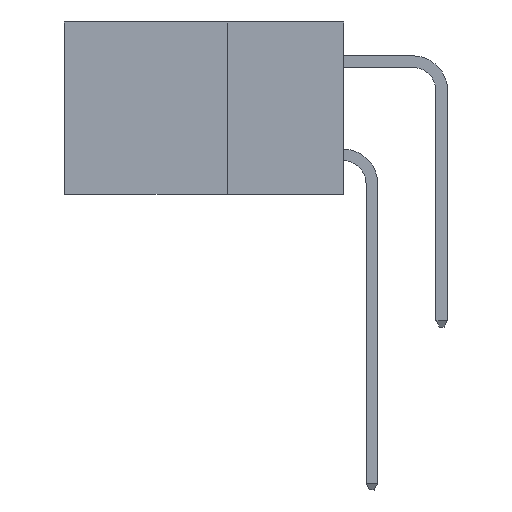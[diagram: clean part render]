
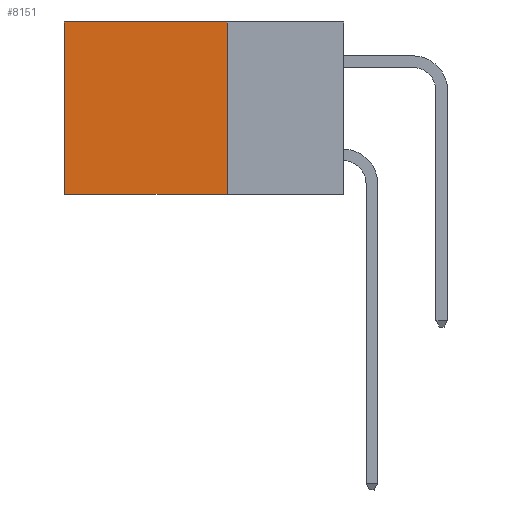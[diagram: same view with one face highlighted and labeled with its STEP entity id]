
A CAD part, left-side view. The second image highlights one B-rep face of the part: STEP entity #8151.
In plain terms, the highlighted planar face has unit normal (-1, 0, 0).
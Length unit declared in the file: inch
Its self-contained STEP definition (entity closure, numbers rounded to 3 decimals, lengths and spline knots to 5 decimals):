
#38 = VERTEX_POINT ( 'NONE', #597 ) ;
#238 = FACE_OUTER_BOUND ( 'NONE', #12392, .T. ) ;
#333 = LINE ( 'NONE', #8152, #9993 ) ;
#480 = CARTESIAN_POINT ( 'NONE',  ( 0.298, 0.6, 0. ) ) ;
#597 = CARTESIAN_POINT ( 'NONE',  ( 0.298, 0.6, -0.37 ) ) ;
#1144 = CARTESIAN_POINT ( 'NONE',  ( 0.298, 0.25, 0. ) ) ;
#1227 = VERTEX_POINT ( 'NONE', #12031 ) ;
#2261 = PLANE ( 'NONE',  #10365 ) ;
#2328 = VERTEX_POINT ( 'NONE', #14279 ) ;
#2749 = VERTEX_POINT ( 'NONE', #480 ) ;
#3270 = EDGE_CURVE ( 'NONE', #1227, #2328, #13689, .T. ) ;
#5617 = DIRECTION ( 'NONE',  ( 0., 0., -1. ) ) ;
#5669 = ORIENTED_EDGE ( 'NONE', *, *, #13952, .T. ) ;
#5700 = DIRECTION ( 'NONE',  ( 0., 0., -1. ) ) ;
#5897 = EDGE_CURVE ( 'NONE', #2749, #38, #11550, .T. ) ;
#7063 = ORIENTED_EDGE ( 'NONE', *, *, #5897, .T. ) ;
#7434 = CARTESIAN_POINT ( 'NONE',  ( 0.298, 0.6, 0. ) ) ;
#8151 = ADVANCED_FACE ( 'NONE', ( #238 ), #2261, .F. ) ;
#8152 = CARTESIAN_POINT ( 'NONE',  ( 0.298, 0.25, 0. ) ) ;
#9119 = DIRECTION ( 'NONE',  ( 0., 1., 0. ) ) ;
#9647 = DIRECTION ( 'NONE',  ( 0., 0., -1. ) ) ;
#9993 = VECTOR ( 'NONE', #12605, 39.37008 ) ;
#10324 = VECTOR ( 'NONE', #9647, 39.37008 ) ;
#10365 = AXIS2_PLACEMENT_3D ( 'NONE', #1144, #11194, #5617 ) ;
#10730 = VECTOR ( 'NONE', #5700, 39.37008 ) ;
#11194 = DIRECTION ( 'NONE',  ( 1., 0., 0. ) ) ;
#11227 = EDGE_CURVE ( 'NONE', #2328, #38, #13574, .T. ) ;
#11403 = CARTESIAN_POINT ( 'NONE',  ( 0.298, 0.25, -0.37 ) ) ;
#11550 = LINE ( 'NONE', #7434, #10324 ) ;
#11661 = VECTOR ( 'NONE', #9119, 39.37008 ) ;
#12031 = CARTESIAN_POINT ( 'NONE',  ( 0.298, 0.25, 0. ) ) ;
#12392 = EDGE_LOOP ( 'NONE', ( #7063, #13327, #14272, #5669 ) ) ;
#12446 = CARTESIAN_POINT ( 'NONE',  ( 0.298, 0.25, 0. ) ) ;
#12605 = DIRECTION ( 'NONE',  ( 0., 1., 0. ) ) ;
#13327 = ORIENTED_EDGE ( 'NONE', *, *, #11227, .F. ) ;
#13574 = LINE ( 'NONE', #11403, #11661 ) ;
#13689 = LINE ( 'NONE', #12446, #10730 ) ;
#13952 = EDGE_CURVE ( 'NONE', #1227, #2749, #333, .T. ) ;
#14272 = ORIENTED_EDGE ( 'NONE', *, *, #3270, .F. ) ;
#14279 = CARTESIAN_POINT ( 'NONE',  ( 0.298, 0.25, -0.37 ) ) ;
